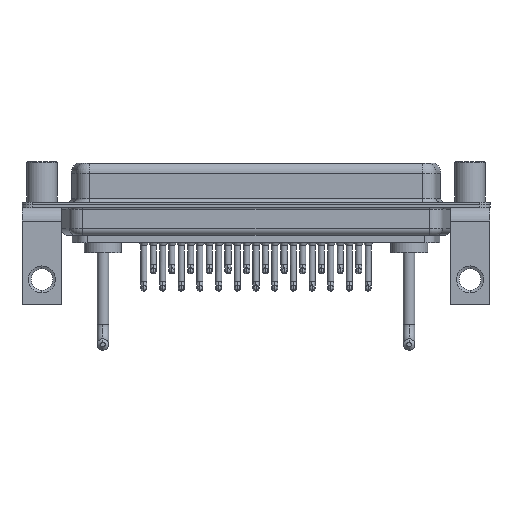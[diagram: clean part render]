
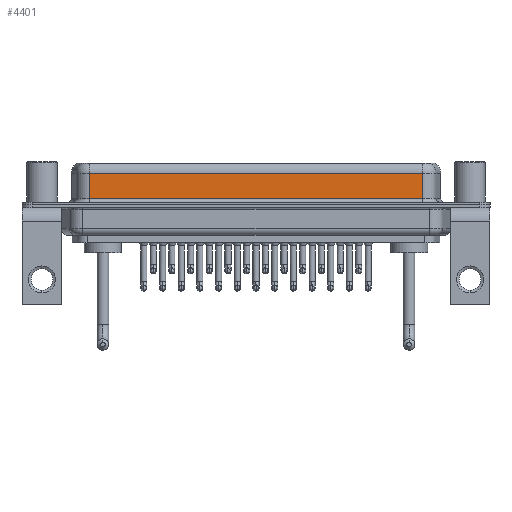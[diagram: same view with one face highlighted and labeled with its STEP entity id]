
A CAD part, front view. The second image highlights one B-rep face of the part: STEP entity #4401.
In plain terms, the highlighted planar face has unit normal (0, -1, 0).
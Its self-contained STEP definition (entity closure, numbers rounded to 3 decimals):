
#828 = DIRECTION ( 'NONE',  ( -1., 0., 0. ) ) ;
#1299 = VECTOR ( 'NONE', #26303, 1000. ) ;
#2148 = LINE ( 'NONE', #10166, #3848 ) ;
#3848 = VECTOR ( 'NONE', #8516, 1000. ) ;
#3957 = CARTESIAN_POINT ( 'NONE',  ( 7.038, -3.95, 0.9 ) ) ;
#4401 = ADVANCED_FACE ( 'NONE', ( #18916 ), #18778, .F. ) ;
#6905 = LINE ( 'NONE', #21700, #19294 ) ;
#7811 = CARTESIAN_POINT ( 'NONE',  ( 7.038, -3.95, 4.65 ) ) ;
#8010 = CARTESIAN_POINT ( 'NONE',  ( 56.462, -3.95, 4.65 ) ) ;
#8299 = AXIS2_PLACEMENT_3D ( 'NONE', #21257, #10739, #10197 ) ;
#8516 = DIRECTION ( 'NONE',  ( 1., 0., 0. ) ) ;
#10166 = CARTESIAN_POINT ( 'NONE',  ( 56.462, -3.95, 0.9 ) ) ;
#10197 = DIRECTION ( 'NONE',  ( 0., 0., 1. ) ) ;
#10739 = DIRECTION ( 'NONE',  ( 0., 1., 0. ) ) ;
#10972 = DIRECTION ( 'NONE',  ( 0., 0., -1. ) ) ;
#11107 = LINE ( 'NONE', #17326, #22276 ) ;
#12586 = ORIENTED_EDGE ( 'NONE', *, *, #14408, .F. ) ;
#14408 = EDGE_CURVE ( 'NONE', #21513, #25326, #11107, .T. ) ;
#16558 = EDGE_CURVE ( 'NONE', #21513, #20532, #6905, .T. ) ;
#17281 = EDGE_CURVE ( 'NONE', #17526, #25326, #2148, .T. ) ;
#17326 = CARTESIAN_POINT ( 'NONE',  ( 56.462, -3.95, 6.4 ) ) ;
#17526 = VERTEX_POINT ( 'NONE', #3957 ) ;
#18778 = PLANE ( 'NONE',  #8299 ) ;
#18916 = FACE_OUTER_BOUND ( 'NONE', #21450, .T. ) ;
#19294 = VECTOR ( 'NONE', #828, 1000. ) ;
#19921 = ORIENTED_EDGE ( 'NONE', *, *, #17281, .T. ) ;
#20532 = VERTEX_POINT ( 'NONE', #7811 ) ;
#20681 = EDGE_CURVE ( 'NONE', #20532, #17526, #22159, .T. ) ;
#21257 = CARTESIAN_POINT ( 'NONE',  ( 56.462, -3.95, 6.4 ) ) ;
#21331 = ORIENTED_EDGE ( 'NONE', *, *, #16558, .T. ) ;
#21450 = EDGE_LOOP ( 'NONE', ( #12586, #21331, #26122, #19921 ) ) ;
#21513 = VERTEX_POINT ( 'NONE', #8010 ) ;
#21700 = CARTESIAN_POINT ( 'NONE',  ( 56.462, -3.95, 4.65 ) ) ;
#22159 = LINE ( 'NONE', #26027, #1299 ) ;
#22276 = VECTOR ( 'NONE', #10972, 1000. ) ;
#22840 = CARTESIAN_POINT ( 'NONE',  ( 56.462, -3.95, 0.9 ) ) ;
#25326 = VERTEX_POINT ( 'NONE', #22840 ) ;
#26027 = CARTESIAN_POINT ( 'NONE',  ( 7.038, -3.95, 6.4 ) ) ;
#26122 = ORIENTED_EDGE ( 'NONE', *, *, #20681, .T. ) ;
#26303 = DIRECTION ( 'NONE',  ( 0., 0., -1. ) ) ;
